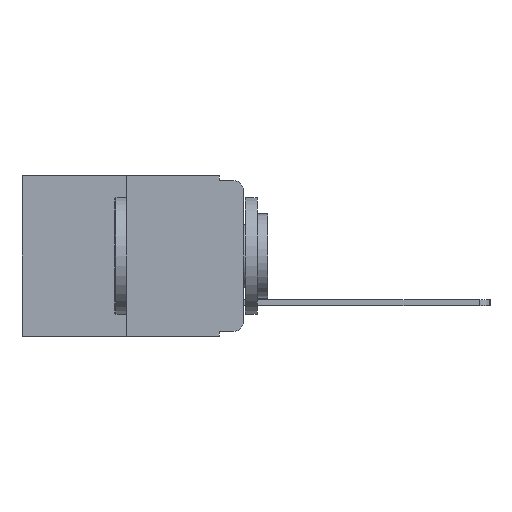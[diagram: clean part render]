
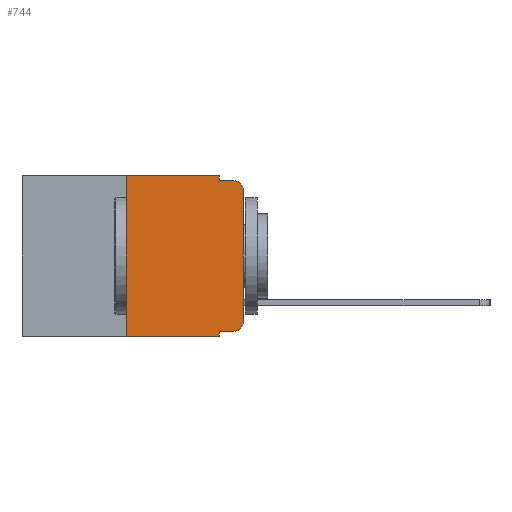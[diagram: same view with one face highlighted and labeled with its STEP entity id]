
A CAD part, left-side view. The second image highlights one B-rep face of the part: STEP entity #744.
In plain terms, the highlighted planar face has unit normal (-1, 0, 0).
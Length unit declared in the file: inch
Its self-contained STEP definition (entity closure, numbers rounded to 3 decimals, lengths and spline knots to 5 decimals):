
#585 = VERTEX_POINT ( 'NONE', #10120 ) ;
#638 = DIRECTION ( 'NONE',  ( 0., 0., -1. ) ) ;
#744 = ADVANCED_FACE ( 'NONE', ( #9001 ), #9260, .F. ) ;
#836 = EDGE_CURVE ( 'NONE', #7486, #10582, #12263, .T. ) ;
#851 = ORIENTED_EDGE ( 'NONE', *, *, #836, .F. ) ;
#1190 = ORIENTED_EDGE ( 'NONE', *, *, #1373, .T. ) ;
#1216 = VERTEX_POINT ( 'NONE', #6986 ) ;
#1296 = VERTEX_POINT ( 'NONE', #3135 ) ;
#1373 = EDGE_CURVE ( 'NONE', #10426, #4349, #9392, .T. ) ;
#1776 = EDGE_CURVE ( 'NONE', #5923, #7486, #8159, .T. ) ;
#1815 = CARTESIAN_POINT ( 'NONE',  ( 0., 0.051, 0. ) ) ;
#1980 = VECTOR ( 'NONE', #5930, 39.37008 ) ;
#2158 = EDGE_CURVE ( 'NONE', #10582, #1296, #9511, .T. ) ;
#2200 = EDGE_CURVE ( 'NONE', #1216, #4733, #4541, .T. ) ;
#2621 = DIRECTION ( 'NONE',  ( 1., 0., 0. ) ) ;
#3001 = VERTEX_POINT ( 'NONE', #11101 ) ;
#3089 = CARTESIAN_POINT ( 'NONE',  ( 0., 0.051, -0.333 ) ) ;
#3135 = CARTESIAN_POINT ( 'NONE',  ( 0., 0.02, -0.01 ) ) ;
#3153 = EDGE_LOOP ( 'NONE', ( #1190, #8299, #9292, #851, #8942, #7402, #9471, #4500, #8240, #8243 ) ) ;
#3183 = CARTESIAN_POINT ( 'NONE',  ( 0., 0.051, 0. ) ) ;
#3740 = LINE ( 'NONE', #4701, #8828 ) ;
#3838 = DIRECTION ( 'NONE',  ( 0., -1., 0. ) ) ;
#3901 = VECTOR ( 'NONE', #3838, 39.37008 ) ;
#4085 = VECTOR ( 'NONE', #9185, 39.37008 ) ;
#4349 = VERTEX_POINT ( 'NONE', #10982 ) ;
#4470 = CARTESIAN_POINT ( 'NONE',  ( 0., 0.25, 0. ) ) ;
#4500 = ORIENTED_EDGE ( 'NONE', *, *, #9325, .F. ) ;
#4541 = LINE ( 'NONE', #9543, #3901 ) ;
#4701 = CARTESIAN_POINT ( 'NONE',  ( 0., 0.25, 0. ) ) ;
#4702 = CIRCLE ( 'NONE', #10592, 0.02 ) ;
#4729 = LINE ( 'NONE', #1815, #1980 ) ;
#4733 = VERTEX_POINT ( 'NONE', #5412 ) ;
#5048 = VECTOR ( 'NONE', #10323, 39.37008 ) ;
#5079 = DIRECTION ( 'NONE',  ( 0., -1., 0. ) ) ;
#5412 = CARTESIAN_POINT ( 'NONE',  ( 0., 0.051, -0.343 ) ) ;
#5471 = CARTESIAN_POINT ( 'NONE',  ( 0., 0.02, -0.313 ) ) ;
#5691 = DIRECTION ( 'NONE',  ( 0., 0., 1. ) ) ;
#5738 = CARTESIAN_POINT ( 'NONE',  ( 0., 0.051, -0.01 ) ) ;
#5798 = CARTESIAN_POINT ( 'NONE',  ( 0., 0., 0. ) ) ;
#5923 = VERTEX_POINT ( 'NONE', #4470 ) ;
#5930 = DIRECTION ( 'NONE',  ( 0., 0., -1. ) ) ;
#5957 = AXIS2_PLACEMENT_3D ( 'NONE', #12057, #6776, #638 ) ;
#6459 = DIRECTION ( 'NONE',  ( 0., 0., -1. ) ) ;
#6776 = DIRECTION ( 'NONE',  ( -1., 0., 0. ) ) ;
#6986 = CARTESIAN_POINT ( 'NONE',  ( 0., 0.25, -0.343 ) ) ;
#7027 = CIRCLE ( 'NONE', #5957, 0.02 ) ;
#7402 = ORIENTED_EDGE ( 'NONE', *, *, #7837, .F. ) ;
#7486 = VERTEX_POINT ( 'NONE', #3183 ) ;
#7837 = EDGE_CURVE ( 'NONE', #1216, #5923, #3740, .T. ) ;
#7899 = CARTESIAN_POINT ( 'NONE',  ( 0., 0.473, 0. ) ) ;
#8098 = CARTESIAN_POINT ( 'NONE',  ( 0., 0.473, 0. ) ) ;
#8159 = LINE ( 'NONE', #7899, #12242 ) ;
#8240 = ORIENTED_EDGE ( 'NONE', *, *, #8804, .T. ) ;
#8243 = ORIENTED_EDGE ( 'NONE', *, *, #10250, .T. ) ;
#8299 = ORIENTED_EDGE ( 'NONE', *, *, #9817, .T. ) ;
#8804 = EDGE_CURVE ( 'NONE', #3001, #585, #11544, .T. ) ;
#8828 = VECTOR ( 'NONE', #5691, 39.37008 ) ;
#8884 = DIRECTION ( 'NONE',  ( 0., -1., 0. ) ) ;
#8942 = ORIENTED_EDGE ( 'NONE', *, *, #1776, .F. ) ;
#9001 = FACE_OUTER_BOUND ( 'NONE', #3153, .T. ) ;
#9185 = DIRECTION ( 'NONE',  ( 0., 0., 1. ) ) ;
#9260 = PLANE ( 'NONE',  #9308 ) ;
#9292 = ORIENTED_EDGE ( 'NONE', *, *, #2158, .F. ) ;
#9308 = AXIS2_PLACEMENT_3D ( 'NONE', #8098, #2621, #9375 ) ;
#9325 = EDGE_CURVE ( 'NONE', #3001, #4733, #4729, .T. ) ;
#9375 = DIRECTION ( 'NONE',  ( 0., 0., -1. ) ) ;
#9392 = LINE ( 'NONE', #5798, #4085 ) ;
#9447 = DIRECTION ( 'NONE',  ( 0., -1., 0. ) ) ;
#9471 = ORIENTED_EDGE ( 'NONE', *, *, #2200, .T. ) ;
#9494 = VECTOR ( 'NONE', #8884, 39.37008 ) ;
#9511 = LINE ( 'NONE', #5738, #11563 ) ;
#9543 = CARTESIAN_POINT ( 'NONE',  ( 0., 0.473, -0.343 ) ) ;
#9817 = EDGE_CURVE ( 'NONE', #4349, #1296, #7027, .T. ) ;
#9874 = CARTESIAN_POINT ( 'NONE',  ( 0., 0.051, 0. ) ) ;
#10120 = CARTESIAN_POINT ( 'NONE',  ( 0., 0.02, -0.333 ) ) ;
#10250 = EDGE_CURVE ( 'NONE', #585, #10426, #4702, .T. ) ;
#10323 = DIRECTION ( 'NONE',  ( 0., 0., -1. ) ) ;
#10426 = VERTEX_POINT ( 'NONE', #11964 ) ;
#10499 = CARTESIAN_POINT ( 'NONE',  ( 0., 0.051, -0.01 ) ) ;
#10582 = VERTEX_POINT ( 'NONE', #10499 ) ;
#10592 = AXIS2_PLACEMENT_3D ( 'NONE', #5471, #11785, #6459 ) ;
#10982 = CARTESIAN_POINT ( 'NONE',  ( 0., 0., -0.03 ) ) ;
#11101 = CARTESIAN_POINT ( 'NONE',  ( 0., 0.051, -0.333 ) ) ;
#11544 = LINE ( 'NONE', #3089, #9494 ) ;
#11563 = VECTOR ( 'NONE', #9447, 39.37008 ) ;
#11785 = DIRECTION ( 'NONE',  ( -1., 0., 0. ) ) ;
#11964 = CARTESIAN_POINT ( 'NONE',  ( 0., 0., -0.313 ) ) ;
#12057 = CARTESIAN_POINT ( 'NONE',  ( 0., 0.02, -0.03 ) ) ;
#12242 = VECTOR ( 'NONE', #5079, 39.37008 ) ;
#12263 = LINE ( 'NONE', #9874, #5048 ) ;
